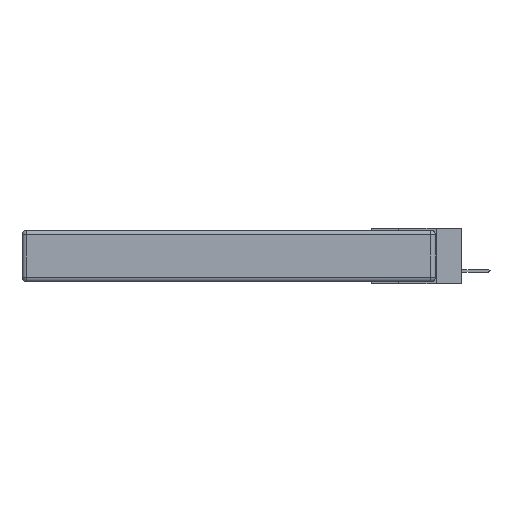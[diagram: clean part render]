
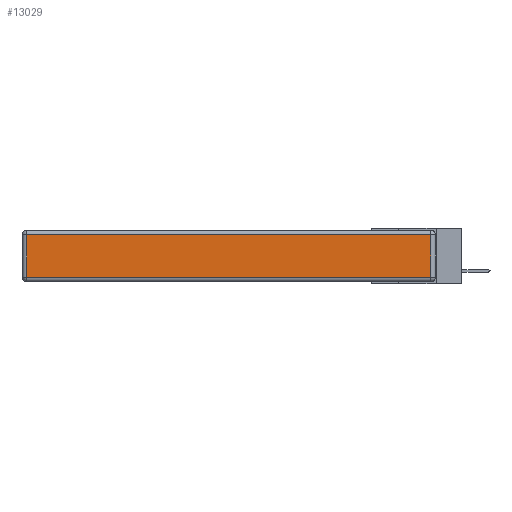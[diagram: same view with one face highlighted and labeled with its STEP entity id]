
A CAD part, left-side view. The second image highlights one B-rep face of the part: STEP entity #13029.
In plain terms, the highlighted planar face has unit normal (-1, 0, 0).
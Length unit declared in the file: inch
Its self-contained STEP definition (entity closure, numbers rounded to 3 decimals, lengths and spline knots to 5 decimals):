
#574 = DIRECTION ( 'NONE',  ( 0., 0., 1. ) ) ;
#1973 = VERTEX_POINT ( 'NONE', #17335 ) ;
#2463 = VERTEX_POINT ( 'NONE', #20640 ) ;
#2681 = DIRECTION ( 'NONE',  ( 0., 0., 1. ) ) ;
#2815 = PLANE ( 'NONE',  #12104 ) ;
#2854 = EDGE_CURVE ( 'NONE', #19653, #2463, #2885, .T. ) ;
#2885 = LINE ( 'NONE', #7315, #18546 ) ;
#4824 = ORIENTED_EDGE ( 'NONE', *, *, #2854, .T. ) ;
#6513 = VECTOR ( 'NONE', #25995, 39.37008 ) ;
#7166 = EDGE_CURVE ( 'NONE', #2463, #22980, #7504, .T. ) ;
#7315 = CARTESIAN_POINT ( 'NONE',  ( 0., 2.75, -0.03 ) ) ;
#7504 = LINE ( 'NONE', #10618, #6513 ) ;
#7804 = EDGE_CURVE ( 'NONE', #1973, #19653, #21411, .T. ) ;
#9015 = EDGE_CURVE ( 'NONE', #22980, #1973, #26146, .T. ) ;
#10618 = CARTESIAN_POINT ( 'NONE',  ( 0., 2.72, -0.343 ) ) ;
#10780 = ORIENTED_EDGE ( 'NONE', *, *, #9015, .T. ) ;
#11251 = VECTOR ( 'NONE', #2681, 39.37008 ) ;
#12104 = AXIS2_PLACEMENT_3D ( 'NONE', #20383, #22294, #574 ) ;
#12927 = ORIENTED_EDGE ( 'NONE', *, *, #7166, .T. ) ;
#13029 = ADVANCED_FACE ( 'NONE', ( #25858 ), #2815, .T. ) ;
#13858 = DIRECTION ( 'NONE',  ( 0., 1., 0. ) ) ;
#15245 = VECTOR ( 'NONE', #25538, 39.37008 ) ;
#15669 = EDGE_LOOP ( 'NONE', ( #10780, #21508, #4824, #12927 ) ) ;
#17335 = CARTESIAN_POINT ( 'NONE',  ( 0., 0.03, -0.313 ) ) ;
#17424 = CARTESIAN_POINT ( 'NONE',  ( 0., 2.72, -0.313 ) ) ;
#18546 = VECTOR ( 'NONE', #13858, 39.37008 ) ;
#19653 = VERTEX_POINT ( 'NONE', #25983 ) ;
#19890 = CARTESIAN_POINT ( 'NONE',  ( 0., 0.03, -0.343 ) ) ;
#20383 = CARTESIAN_POINT ( 'NONE',  ( 0., 0., -0.343 ) ) ;
#20640 = CARTESIAN_POINT ( 'NONE',  ( 0., 2.72, -0.03 ) ) ;
#21411 = LINE ( 'NONE', #19890, #11251 ) ;
#21508 = ORIENTED_EDGE ( 'NONE', *, *, #7804, .T. ) ;
#22294 = DIRECTION ( 'NONE',  ( -1., 0., 0. ) ) ;
#22980 = VERTEX_POINT ( 'NONE', #17424 ) ;
#23444 = CARTESIAN_POINT ( 'NONE',  ( 0., 0., -0.313 ) ) ;
#25538 = DIRECTION ( 'NONE',  ( 0., -1., 0. ) ) ;
#25858 = FACE_OUTER_BOUND ( 'NONE', #15669, .T. ) ;
#25983 = CARTESIAN_POINT ( 'NONE',  ( 0., 0.03, -0.03 ) ) ;
#25995 = DIRECTION ( 'NONE',  ( 0., 0., -1. ) ) ;
#26146 = LINE ( 'NONE', #23444, #15245 ) ;
